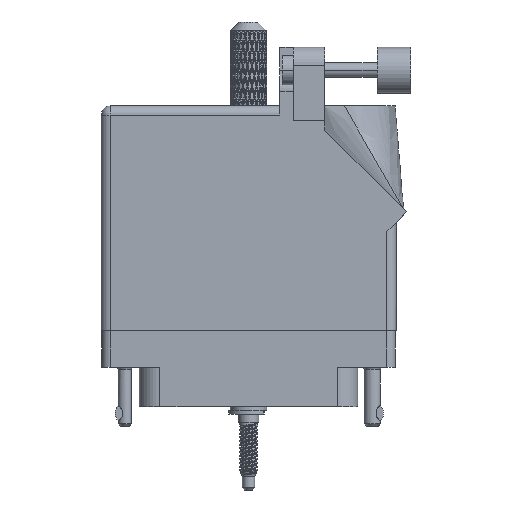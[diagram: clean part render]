
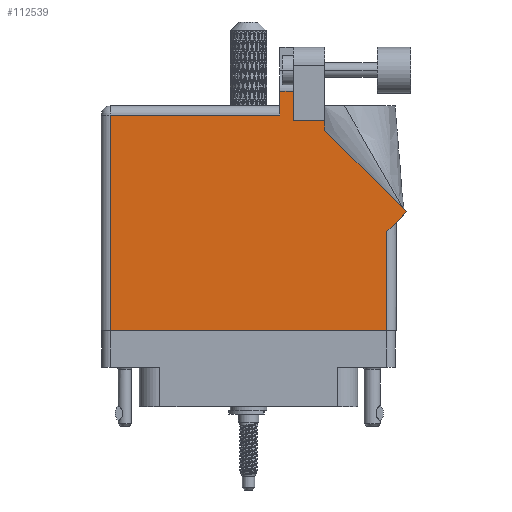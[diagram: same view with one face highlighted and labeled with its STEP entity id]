
A CAD part, front view. The second image highlights one B-rep face of the part: STEP entity #112539.
In plain terms, the highlighted face is planar.
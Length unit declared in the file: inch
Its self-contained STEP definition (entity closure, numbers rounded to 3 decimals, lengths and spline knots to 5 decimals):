
#2213 = VERTEX_POINT ( 'NONE', #93330 ) ;
#6910 = VERTEX_POINT ( 'NONE', #49806 ) ;
#8343 = VERTEX_POINT ( 'NONE', #82761 ) ;
#9027 = EDGE_CURVE ( 'NONE', #20042, #6910, #67213, .T. ) ;
#10022 = EDGE_CURVE ( 'NONE', #20432, #24844, #103950, .T. ) ;
#12344 = VECTOR ( 'NONE', #84381, 39.37008 ) ;
#15179 = LINE ( 'NONE', #66519, #12344 ) ;
#15563 = DIRECTION ( 'NONE',  ( -1., 0., 0. ) ) ;
#18558 = ORIENTED_EDGE ( 'NONE', *, *, #105708, .T. ) ;
#20042 = VERTEX_POINT ( 'NONE', #105803 ) ;
#20432 = VERTEX_POINT ( 'NONE', #29278 ) ;
#20991 = CARTESIAN_POINT ( 'NONE',  ( 0.306, 1.33, 0.455 ) ) ;
#23196 = CARTESIAN_POINT ( 'NONE',  ( 0.212, 1.5315, 0.455 ) ) ;
#24538 = DIRECTION ( 'NONE',  ( 0., -1., 0. ) ) ;
#24844 = VERTEX_POINT ( 'NONE', #23196 ) ;
#29278 = CARTESIAN_POINT ( 'NONE',  ( 0.306, 1.5315, 0.455 ) ) ;
#30466 = LINE ( 'NONE', #85957, #51499 ) ;
#31627 = DIRECTION ( 'NONE',  ( -1., 0., 0. ) ) ;
#33089 = ORIENTED_EDGE ( 'NONE', *, *, #37993, .T. ) ;
#35552 = VECTOR ( 'NONE', #36162, 39.37008 ) ;
#35929 = EDGE_CURVE ( 'NONE', #8343, #87829, #67365, .T. ) ;
#36162 = DIRECTION ( 'NONE',  ( -1., 0., 0. ) ) ;
#36179 = VECTOR ( 'NONE', #65380, 39.37008 ) ;
#37851 = VECTOR ( 'NONE', #84677, 39.37008 ) ;
#37993 = EDGE_CURVE ( 'NONE', #6910, #72873, #101806, .T. ) ;
#38670 = CARTESIAN_POINT ( 'NONE',  ( 0.943, 0.575, 0.455 ) ) ;
#39369 = CARTESIAN_POINT ( 'NONE',  ( 0.519, 1.33, 0.455 ) ) ;
#39503 = CARTESIAN_POINT ( 'NONE',  ( -1.005, -0.1, 0.455 ) ) ;
#41857 = ORIENTED_EDGE ( 'NONE', *, *, #43467, .T. ) ;
#42331 = DIRECTION ( 'NONE',  ( 0., 1., 0. ) ) ;
#42336 = ORIENTED_EDGE ( 'NONE', *, *, #113026, .T. ) ;
#43467 = EDGE_CURVE ( 'NONE', #87829, #107526, #72060, .T. ) ;
#44791 = CARTESIAN_POINT ( 'NONE',  ( 0.63677, 1.5315, 0.455 ) ) ;
#46058 = VERTEX_POINT ( 'NONE', #38670 ) ;
#46714 = CARTESIAN_POINT ( 'NONE',  ( 0.212, 1.43, 0.455 ) ) ;
#47023 = DIRECTION ( 'NONE',  ( 0., 1., 0. ) ) ;
#47407 = CARTESIAN_POINT ( 'NONE',  ( 0.519, 1.26442, 0.455 ) ) ;
#49806 = CARTESIAN_POINT ( 'NONE',  ( 0.519, 1.26442, 0.455 ) ) ;
#51004 = VECTOR ( 'NONE', #102614, 39.37008 ) ;
#51499 = VECTOR ( 'NONE', #42331, 39.37008 ) ;
#51833 = EDGE_CURVE ( 'NONE', #24844, #2213, #83597, .T. ) ;
#52048 = EDGE_CURVE ( 'NONE', #107526, #46058, #30466, .T. ) ;
#52255 = CARTESIAN_POINT ( 'NONE',  ( -0.943, -0.1, 0.455 ) ) ;
#53904 = ORIENTED_EDGE ( 'NONE', *, *, #52048, .T. ) ;
#56227 = VECTOR ( 'NONE', #67028, 39.37008 ) ;
#57884 = CARTESIAN_POINT ( 'NONE',  ( 1.07571, 0.70771, 0.455 ) ) ;
#58439 = CARTESIAN_POINT ( 'NONE',  ( -1.005, 1.368, 0.455 ) ) ;
#59381 = LINE ( 'NONE', #112349, #51004 ) ;
#59400 = CARTESIAN_POINT ( 'NONE',  ( -0.943, -0.1, 0.455 ) ) ;
#59776 = EDGE_CURVE ( 'NONE', #72873, #89813, #59381, .T. ) ;
#63714 = VECTOR ( 'NONE', #111660, 39.37008 ) ;
#65380 = DIRECTION ( 'NONE',  ( 0., -1., 0. ) ) ;
#66519 = CARTESIAN_POINT ( 'NONE',  ( 0.306, 1.33, 0.455 ) ) ;
#66788 = DIRECTION ( 'NONE',  ( 0., 0., -1. ) ) ;
#67028 = DIRECTION ( 'NONE',  ( 0.707, 0.707, 0. ) ) ;
#67213 = LINE ( 'NONE', #57884, #37851 ) ;
#67365 = LINE ( 'NONE', #52255, #88210 ) ;
#69597 = EDGE_CURVE ( 'NONE', #2213, #8343, #87880, .T. ) ;
#69616 = EDGE_LOOP ( 'NONE', ( #18558, #102629, #103164, #72042, #103165, #41857, #53904, #42336, #79811, #33089, #113735 ) ) ;
#72042 = ORIENTED_EDGE ( 'NONE', *, *, #69597, .T. ) ;
#72060 = LINE ( 'NONE', #39503, #63714 ) ;
#72873 = VERTEX_POINT ( 'NONE', #39369 ) ;
#79811 = ORIENTED_EDGE ( 'NONE', *, *, #9027, .T. ) ;
#80882 = VECTOR ( 'NONE', #47023, 39.37008 ) ;
#82761 = CARTESIAN_POINT ( 'NONE',  ( -0.943, 1.368, 0.455 ) ) ;
#83597 = LINE ( 'NONE', #46714, #36179 ) ;
#84381 = DIRECTION ( 'NONE',  ( 0., 1., 0. ) ) ;
#84677 = DIRECTION ( 'NONE',  ( -0.707, 0.707, 0. ) ) ;
#85957 = CARTESIAN_POINT ( 'NONE',  ( 0.943, 0.637, 0.455 ) ) ;
#86174 = PLANE ( 'NONE',  #101151 ) ;
#87829 = VERTEX_POINT ( 'NONE', #59400 ) ;
#87880 = LINE ( 'NONE', #58439, #90660 ) ;
#88210 = VECTOR ( 'NONE', #24538, 39.37008 ) ;
#89813 = VERTEX_POINT ( 'NONE', #20991 ) ;
#90660 = VECTOR ( 'NONE', #15563, 39.37008 ) ;
#93099 = CARTESIAN_POINT ( 'NONE',  ( 1.005, 0.637, 0.455 ) ) ;
#93330 = CARTESIAN_POINT ( 'NONE',  ( 0.212, 1.368, 0.455 ) ) ;
#96562 = LINE ( 'NONE', #93099, #56227 ) ;
#97510 = CARTESIAN_POINT ( 'NONE',  ( 0.943, -0.1, 0.455 ) ) ;
#101151 = AXIS2_PLACEMENT_3D ( 'NONE', #103006, #66788, #31627 ) ;
#101806 = LINE ( 'NONE', #47407, #80882 ) ;
#102399 = FACE_OUTER_BOUND ( 'NONE', #69616, .T. ) ;
#102614 = DIRECTION ( 'NONE',  ( -1., 0., 0. ) ) ;
#102629 = ORIENTED_EDGE ( 'NONE', *, *, #10022, .T. ) ;
#103006 = CARTESIAN_POINT ( 'NONE',  ( -1.005, 1.43, 0.455 ) ) ;
#103164 = ORIENTED_EDGE ( 'NONE', *, *, #51833, .T. ) ;
#103165 = ORIENTED_EDGE ( 'NONE', *, *, #35929, .T. ) ;
#103950 = LINE ( 'NONE', #44791, #35552 ) ;
#105708 = EDGE_CURVE ( 'NONE', #89813, #20432, #15179, .T. ) ;
#105803 = CARTESIAN_POINT ( 'NONE',  ( 1.07571, 0.70771, 0.455 ) ) ;
#107526 = VERTEX_POINT ( 'NONE', #97510 ) ;
#111660 = DIRECTION ( 'NONE',  ( 1., 0., 0. ) ) ;
#112349 = CARTESIAN_POINT ( 'NONE',  ( 0.519, 1.33, 0.455 ) ) ;
#112539 = ADVANCED_FACE ( 'NONE', ( #102399 ), #86174, .F. ) ;
#113026 = EDGE_CURVE ( 'NONE', #46058, #20042, #96562, .T. ) ;
#113735 = ORIENTED_EDGE ( 'NONE', *, *, #59776, .T. ) ;
